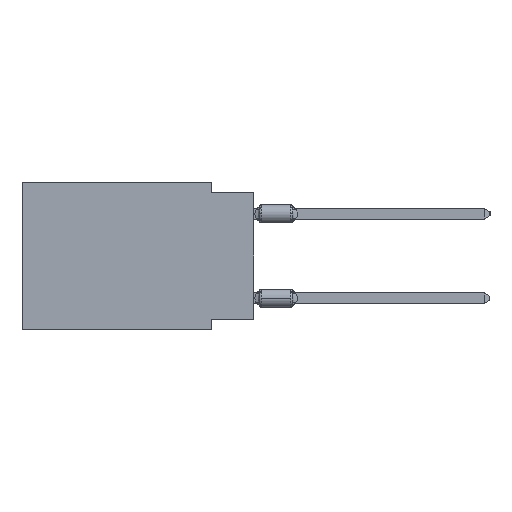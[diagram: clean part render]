
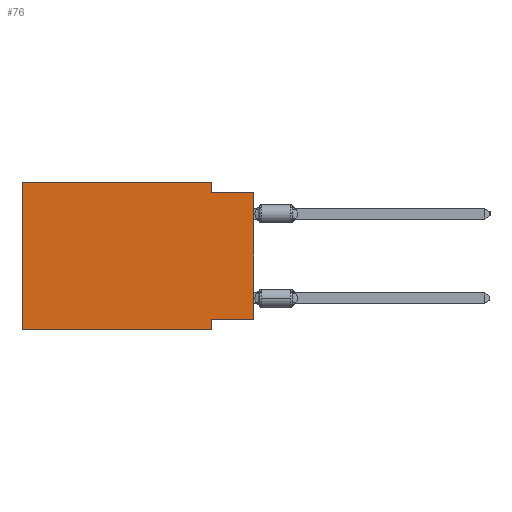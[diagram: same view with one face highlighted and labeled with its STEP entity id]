
A CAD part, left-side view. The second image highlights one B-rep face of the part: STEP entity #76.
In plain terms, the highlighted planar face has unit normal (-1, 0, 0).
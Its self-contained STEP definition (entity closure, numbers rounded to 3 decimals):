
#76 = ADVANCED_FACE ( 'NONE', ( #4669 ), #12964, .F. ) ;
#185 = CARTESIAN_POINT ( 'NONE',  ( 0., 2.54, 0. ) ) ;
#1074 = LINE ( 'NONE', #5705, #20475 ) ;
#1161 = DIRECTION ( 'NONE',  ( 0., 0., -1. ) ) ;
#1592 = VERTEX_POINT ( 'NONE', #185 ) ;
#2479 = EDGE_CURVE ( 'NONE', #21535, #11016, #19917, .T. ) ;
#3118 = EDGE_CURVE ( 'NONE', #12755, #17422, #20027, .T. ) ;
#3171 = VECTOR ( 'NONE', #3850, 1000. ) ;
#3710 = CARTESIAN_POINT ( 'NONE',  ( 0., 0., 0. ) ) ;
#3850 = DIRECTION ( 'NONE',  ( 0., 0., 1. ) ) ;
#4568 = EDGE_LOOP ( 'NONE', ( #13788, #14921, #15242, #4765, #22600, #12676, #23099, #8011 ) ) ;
#4669 = FACE_OUTER_BOUND ( 'NONE', #4568, .T. ) ;
#4765 = ORIENTED_EDGE ( 'NONE', *, *, #14788, .F. ) ;
#4887 = CARTESIAN_POINT ( 'NONE',  ( 0., 0., -0.635 ) ) ;
#4985 = CARTESIAN_POINT ( 'NONE',  ( 0., 13.97, -8.89 ) ) ;
#5705 = CARTESIAN_POINT ( 'NONE',  ( 0., 13.97, 0. ) ) ;
#5770 = DIRECTION ( 'NONE',  ( 0., 1., 0. ) ) ;
#5783 = CARTESIAN_POINT ( 'NONE',  ( 0., 2.54, -0.635 ) ) ;
#5908 = VECTOR ( 'NONE', #13452, 1000. ) ;
#6359 = DIRECTION ( 'NONE',  ( 1., 0., 0. ) ) ;
#6464 = CARTESIAN_POINT ( 'NONE',  ( 0., 13.97, 0. ) ) ;
#7057 = VECTOR ( 'NONE', #15418, 1000. ) ;
#7062 = CARTESIAN_POINT ( 'NONE',  ( 0., 2.54, 0. ) ) ;
#7792 = DIRECTION ( 'NONE',  ( 0., 0., 1. ) ) ;
#7793 = AXIS2_PLACEMENT_3D ( 'NONE', #19844, #6359, #17598 ) ;
#8011 = ORIENTED_EDGE ( 'NONE', *, *, #27056, .F. ) ;
#8014 = EDGE_CURVE ( 'NONE', #18633, #11016, #27342, .T. ) ;
#8370 = VECTOR ( 'NONE', #5770, 1000. ) ;
#8938 = CARTESIAN_POINT ( 'NONE',  ( 0., 13.97, 0. ) ) ;
#9087 = LINE ( 'NONE', #15567, #20217 ) ;
#11016 = VERTEX_POINT ( 'NONE', #13488 ) ;
#11292 = DIRECTION ( 'NONE',  ( 0., 0., -1. ) ) ;
#12676 = ORIENTED_EDGE ( 'NONE', *, *, #23402, .T. ) ;
#12755 = VERTEX_POINT ( 'NONE', #22328 ) ;
#12964 = PLANE ( 'NONE',  #7793 ) ;
#13363 = EDGE_CURVE ( 'NONE', #13531, #14409, #1074, .T. ) ;
#13452 = DIRECTION ( 'NONE',  ( 0., -1., 0. ) ) ;
#13488 = CARTESIAN_POINT ( 'NONE',  ( 0., 0., -0.635 ) ) ;
#13508 = VECTOR ( 'NONE', #11292, 1000. ) ;
#13531 = VERTEX_POINT ( 'NONE', #4985 ) ;
#13788 = ORIENTED_EDGE ( 'NONE', *, *, #8014, .T. ) ;
#14409 = VERTEX_POINT ( 'NONE', #6464 ) ;
#14788 = EDGE_CURVE ( 'NONE', #14409, #1592, #19366, .T. ) ;
#14921 = ORIENTED_EDGE ( 'NONE', *, *, #2479, .F. ) ;
#15242 = ORIENTED_EDGE ( 'NONE', *, *, #25277, .F. ) ;
#15418 = DIRECTION ( 'NONE',  ( 0., -1., 0. ) ) ;
#15567 = CARTESIAN_POINT ( 'NONE',  ( 0., 13.97, -8.89 ) ) ;
#16308 = LINE ( 'NONE', #18414, #8370 ) ;
#17422 = VERTEX_POINT ( 'NONE', #27028 ) ;
#17598 = DIRECTION ( 'NONE',  ( 0., 0., -1. ) ) ;
#18414 = CARTESIAN_POINT ( 'NONE',  ( 0., 0., -8.255 ) ) ;
#18633 = VERTEX_POINT ( 'NONE', #20694 ) ;
#19366 = LINE ( 'NONE', #8938, #7057 ) ;
#19844 = CARTESIAN_POINT ( 'NONE',  ( 0., 13.97, 0. ) ) ;
#19917 = LINE ( 'NONE', #4887, #5908 ) ;
#20027 = LINE ( 'NONE', #22665, #22551 ) ;
#20217 = VECTOR ( 'NONE', #26402, 1000. ) ;
#20286 = LINE ( 'NONE', #7062, #13508 ) ;
#20475 = VECTOR ( 'NONE', #7792, 1000. ) ;
#20694 = CARTESIAN_POINT ( 'NONE',  ( 0., 0., -8.255 ) ) ;
#21535 = VERTEX_POINT ( 'NONE', #5783 ) ;
#22328 = CARTESIAN_POINT ( 'NONE',  ( 0., 2.54, -8.255 ) ) ;
#22551 = VECTOR ( 'NONE', #1161, 1000. ) ;
#22600 = ORIENTED_EDGE ( 'NONE', *, *, #13363, .F. ) ;
#22665 = CARTESIAN_POINT ( 'NONE',  ( 0., 2.54, -8.89 ) ) ;
#23099 = ORIENTED_EDGE ( 'NONE', *, *, #3118, .F. ) ;
#23402 = EDGE_CURVE ( 'NONE', #13531, #17422, #9087, .T. ) ;
#25277 = EDGE_CURVE ( 'NONE', #1592, #21535, #20286, .T. ) ;
#26402 = DIRECTION ( 'NONE',  ( 0., -1., 0. ) ) ;
#27028 = CARTESIAN_POINT ( 'NONE',  ( 0., 2.54, -8.89 ) ) ;
#27056 = EDGE_CURVE ( 'NONE', #18633, #12755, #16308, .T. ) ;
#27342 = LINE ( 'NONE', #3710, #3171 ) ;
